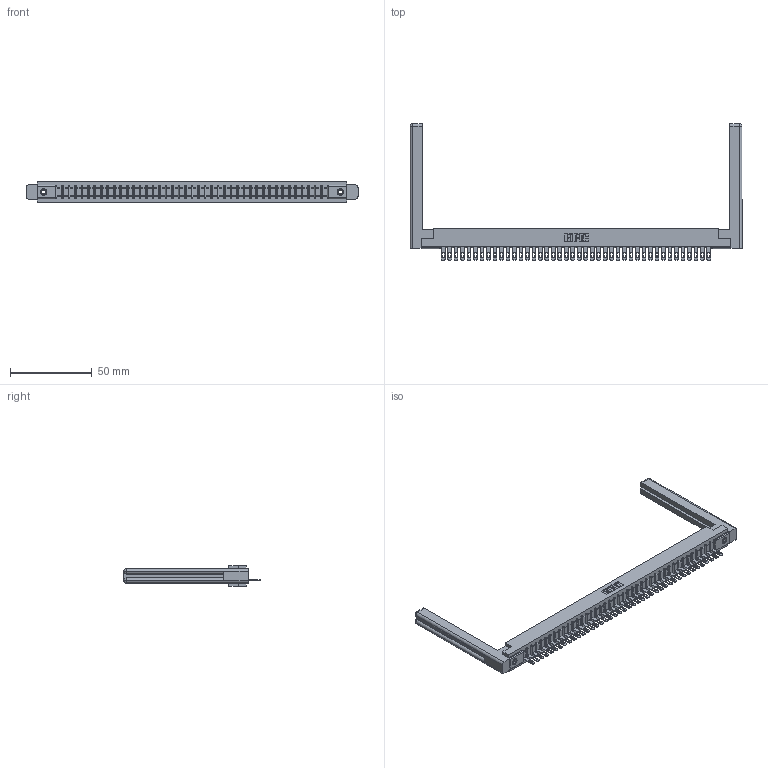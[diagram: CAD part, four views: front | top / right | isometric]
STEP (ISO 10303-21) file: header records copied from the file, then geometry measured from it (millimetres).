
FILE_DESCRIPTION (( 'STEP AP203' ), '1' );
FILE_NAME ('307-042-505-158.STEP', '2019-09-04T07:31:34', ( '' ), ( '' ), 'SwSTEP 2.0', 'SolidWorks 2016', '' );
FILE_SCHEMA (( 'CONFIG_CONTROL_DESIGN' ));
Length unit declared in the file: inch
Products named in the file (5): 307-290-001_505; 307 Part_.156 Dia Mounting Holes; 307-220-058; 345-250-001_345-250-001-102; 307-042-505-158
Assembly tree (47 placements, depth 2):
  307-042-505-158
    307 Part_.156 Dia Mounting Holes
    307-290-001_505  x42
    307-220-058  x2
    345-250-001_345-250-001-102  x2
Bounding box: 203.05 x 83.49 x 12.7 mm (x, y, z)
Volume: 28299.6 mm3; surface area: 27907.4 mm2
Topology: 47 solids, 47 shells, 2655 faces, 7481 edges, 4802 vertices
Faces by surface type: plane 1666, cylinder 879, sphere 86, torus 12, cone 12
Entity records: 38613 total; most frequent: CARTESIAN_POINT 6511, ORIENTED_EDGE 6436, DIRECTION 6294, EDGE_CURVE 3218, VECTOR 2464, LINE 2464, VERTEX_POINT 2078, AXIS2_PLACEMENT_3D 1915
